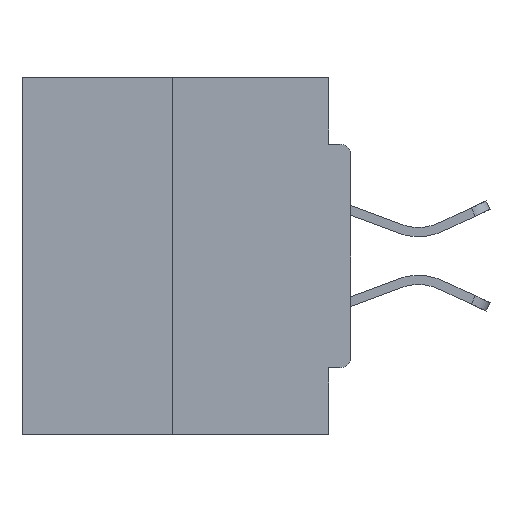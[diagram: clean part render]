
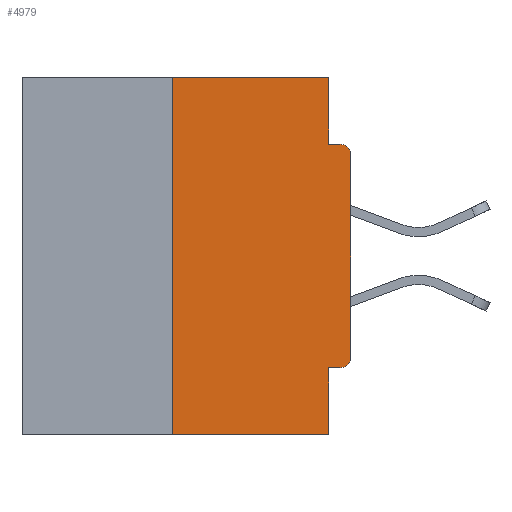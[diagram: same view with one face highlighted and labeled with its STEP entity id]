
A CAD part, left-side view. The second image highlights one B-rep face of the part: STEP entity #4979.
In plain terms, the highlighted planar face has unit normal (-1, 0, 0).
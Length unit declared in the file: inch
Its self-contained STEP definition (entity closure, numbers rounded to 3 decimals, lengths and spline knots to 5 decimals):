
#323 = DIRECTION ( 'NONE',  ( 0., 0., 1. ) ) ;
#2321 = DIRECTION ( 'NONE',  ( 0., 1., 0. ) ) ;
#2807 = DIRECTION ( 'NONE',  ( -1., 0., 0. ) ) ;
#2908 = CARTESIAN_POINT ( 'NONE',  ( 0., 0.015, -0.1085 ) ) ;
#3025 = LINE ( 'NONE', #16205, #9306 ) ;
#3739 = DIRECTION ( 'NONE',  ( 0., 0., -1. ) ) ;
#3919 = EDGE_CURVE ( 'NONE', #10872, #6952, #29535, .T. ) ;
#3934 = VECTOR ( 'NONE', #14271, 39.37008 ) ;
#4979 = ADVANCED_FACE ( 'NONE', ( #32639 ), #22866, .F. ) ;
#4994 = ORIENTED_EDGE ( 'NONE', *, *, #5876, .T. ) ;
#5291 = DIRECTION ( 'NONE',  ( 0., 0., -1. ) ) ;
#5431 = DIRECTION ( 'NONE',  ( 1., 0., 0. ) ) ;
#5876 = EDGE_CURVE ( 'NONE', #14312, #10872, #18267, .T. ) ;
#6662 = DIRECTION ( 'NONE',  ( 0., 0., 1. ) ) ;
#6847 = VECTOR ( 'NONE', #17209, 39.37008 ) ;
#6890 = ORIENTED_EDGE ( 'NONE', *, *, #3919, .T. ) ;
#6952 = VERTEX_POINT ( 'NONE', #21385 ) ;
#6953 = EDGE_CURVE ( 'NONE', #19356, #14886, #32165, .T. ) ;
#7107 = LINE ( 'NONE', #32521, #8287 ) ;
#7473 = ORIENTED_EDGE ( 'NONE', *, *, #6953, .F. ) ;
#8287 = VECTOR ( 'NONE', #2321, 39.37008 ) ;
#8413 = DIRECTION ( 'NONE',  ( 0., 0., -1. ) ) ;
#9074 = CARTESIAN_POINT ( 'NONE',  ( 0., 0.031, -0.4065 ) ) ;
#9306 = VECTOR ( 'NONE', #6662, 39.37008 ) ;
#10503 = DIRECTION ( 'NONE',  ( 0., 0., -1. ) ) ;
#10872 = VERTEX_POINT ( 'NONE', #30227 ) ;
#11692 = VERTEX_POINT ( 'NONE', #30188 ) ;
#11947 = VERTEX_POINT ( 'NONE', #28878 ) ;
#11984 = VECTOR ( 'NONE', #29037, 39.37008 ) ;
#12347 = CARTESIAN_POINT ( 'NONE',  ( 0., 0.031, -0.5 ) ) ;
#12964 = ORIENTED_EDGE ( 'NONE', *, *, #28838, .T. ) ;
#13207 = EDGE_CURVE ( 'NONE', #11692, #25222, #16908, .T. ) ;
#14209 = ORIENTED_EDGE ( 'NONE', *, *, #20255, .F. ) ;
#14271 = DIRECTION ( 'NONE',  ( 0., -1., 0. ) ) ;
#14312 = VERTEX_POINT ( 'NONE', #21294 ) ;
#14673 = CARTESIAN_POINT ( 'NONE',  ( 0., 0.46, -0.5 ) ) ;
#14886 = VERTEX_POINT ( 'NONE', #26547 ) ;
#15775 = ORIENTED_EDGE ( 'NONE', *, *, #24998, .F. ) ;
#16205 = CARTESIAN_POINT ( 'NONE',  ( 0., 0.25, 0. ) ) ;
#16748 = CARTESIAN_POINT ( 'NONE',  ( 0., 0.015, -0.0935 ) ) ;
#16809 = VERTEX_POINT ( 'NONE', #9074 ) ;
#16908 = LINE ( 'NONE', #29432, #3934 ) ;
#17112 = ORIENTED_EDGE ( 'NONE', *, *, #21390, .F. ) ;
#17209 = DIRECTION ( 'NONE',  ( 0., -1., 0. ) ) ;
#18267 = CIRCLE ( 'NONE', #24530, 0.015 ) ;
#18463 = ORIENTED_EDGE ( 'NONE', *, *, #13207, .F. ) ;
#19356 = VERTEX_POINT ( 'NONE', #31507 ) ;
#19841 = LINE ( 'NONE', #14673, #6847 ) ;
#19906 = CIRCLE ( 'NONE', #22991, 0.015 ) ;
#20235 = CARTESIAN_POINT ( 'NONE',  ( 0., 0.031, -0.5 ) ) ;
#20255 = EDGE_CURVE ( 'NONE', #16809, #21033, #22256, .T. ) ;
#20504 = CARTESIAN_POINT ( 'NONE',  ( 0., 0.46, 0. ) ) ;
#20511 = CARTESIAN_POINT ( 'NONE',  ( 0., 0., 0. ) ) ;
#21033 = VERTEX_POINT ( 'NONE', #20235 ) ;
#21294 = CARTESIAN_POINT ( 'NONE',  ( 0., 0.015, -0.4065 ) ) ;
#21385 = CARTESIAN_POINT ( 'NONE',  ( 0., 0., -0.1085 ) ) ;
#21390 = EDGE_CURVE ( 'NONE', #11947, #19356, #3025, .T. ) ;
#22098 = LINE ( 'NONE', #23844, #29229 ) ;
#22176 = DIRECTION ( 'NONE',  ( 0., 0., -1. ) ) ;
#22256 = LINE ( 'NONE', #12347, #31742 ) ;
#22866 = PLANE ( 'NONE',  #23647 ) ;
#22991 = AXIS2_PLACEMENT_3D ( 'NONE', #2908, #2807, #5291 ) ;
#23647 = AXIS2_PLACEMENT_3D ( 'NONE', #20504, #5431, #10503 ) ;
#23844 = CARTESIAN_POINT ( 'NONE',  ( 0., 0.031, 0. ) ) ;
#24063 = CARTESIAN_POINT ( 'NONE',  ( 0., 0.46, 0. ) ) ;
#24530 = AXIS2_PLACEMENT_3D ( 'NONE', #29209, #31760, #3739 ) ;
#24998 = EDGE_CURVE ( 'NONE', #14886, #11692, #22098, .T. ) ;
#25222 = VERTEX_POINT ( 'NONE', #16748 ) ;
#25235 = ORIENTED_EDGE ( 'NONE', *, *, #26704, .F. ) ;
#26343 = VECTOR ( 'NONE', #323, 39.37008 ) ;
#26547 = CARTESIAN_POINT ( 'NONE',  ( 0., 0.031, 0. ) ) ;
#26704 = EDGE_CURVE ( 'NONE', #14312, #16809, #7107, .T. ) ;
#27933 = EDGE_LOOP ( 'NONE', ( #7473, #17112, #28759, #14209, #25235, #4994, #6890, #12964, #18463, #15775 ) ) ;
#28759 = ORIENTED_EDGE ( 'NONE', *, *, #30041, .T. ) ;
#28838 = EDGE_CURVE ( 'NONE', #6952, #25222, #19906, .T. ) ;
#28878 = CARTESIAN_POINT ( 'NONE',  ( 0., 0.25, -0.5 ) ) ;
#29037 = DIRECTION ( 'NONE',  ( 0., -1., 0. ) ) ;
#29209 = CARTESIAN_POINT ( 'NONE',  ( 0., 0.015, -0.3915 ) ) ;
#29229 = VECTOR ( 'NONE', #8413, 39.37008 ) ;
#29432 = CARTESIAN_POINT ( 'NONE',  ( 0., 0., -0.0935 ) ) ;
#29535 = LINE ( 'NONE', #20511, #26343 ) ;
#30041 = EDGE_CURVE ( 'NONE', #11947, #21033, #19841, .T. ) ;
#30188 = CARTESIAN_POINT ( 'NONE',  ( 0., 0.031, -0.0935 ) ) ;
#30227 = CARTESIAN_POINT ( 'NONE',  ( 0., 0., -0.3915 ) ) ;
#31507 = CARTESIAN_POINT ( 'NONE',  ( 0., 0.25, 0. ) ) ;
#31742 = VECTOR ( 'NONE', #22176, 39.37008 ) ;
#31760 = DIRECTION ( 'NONE',  ( -1., 0., 0. ) ) ;
#32165 = LINE ( 'NONE', #24063, #11984 ) ;
#32521 = CARTESIAN_POINT ( 'NONE',  ( 0., 0., -0.4065 ) ) ;
#32639 = FACE_OUTER_BOUND ( 'NONE', #27933, .T. ) ;
